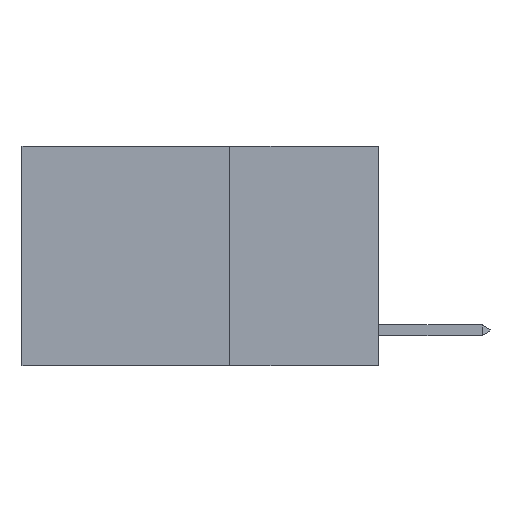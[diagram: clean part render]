
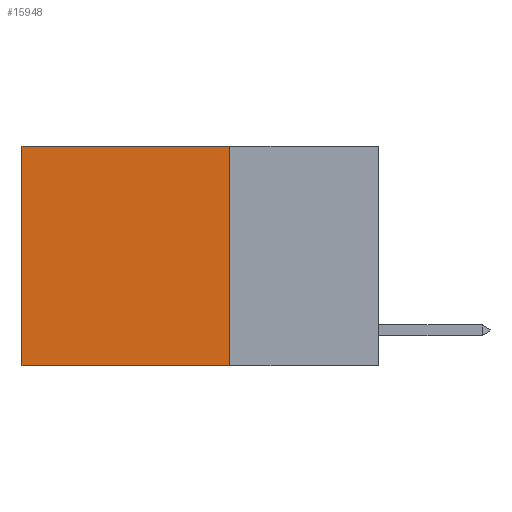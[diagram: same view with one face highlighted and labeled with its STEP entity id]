
A CAD part, left-side view. The second image highlights one B-rep face of the part: STEP entity #15948.
In plain terms, the highlighted planar face has unit normal (-1, 0, 0).
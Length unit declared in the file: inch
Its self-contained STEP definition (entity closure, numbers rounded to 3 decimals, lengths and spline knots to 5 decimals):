
#190 = CARTESIAN_POINT ( 'NONE',  ( 0.2625, 0.25, 0. ) ) ;
#525 = CARTESIAN_POINT ( 'NONE',  ( 0.2625, 0.25, -0.37 ) ) ;
#904 = VECTOR ( 'NONE', #7084, 39.37008 ) ;
#969 = EDGE_CURVE ( 'NONE', #13301, #1964, #5010, .T. ) ;
#1018 = LINE ( 'NONE', #3613, #14707 ) ;
#1738 = CARTESIAN_POINT ( 'NONE',  ( 0.2625, 0.6, -0.37 ) ) ;
#1964 = VERTEX_POINT ( 'NONE', #6426 ) ;
#2545 = PLANE ( 'NONE',  #9981 ) ;
#3000 = DIRECTION ( 'NONE',  ( 0., 0., -1. ) ) ;
#3613 = CARTESIAN_POINT ( 'NONE',  ( 0.2625, 0.6, 0. ) ) ;
#3957 = ORIENTED_EDGE ( 'NONE', *, *, #7245, .F. ) ;
#4469 = EDGE_CURVE ( 'NONE', #13301, #7602, #16827, .T. ) ;
#4696 = EDGE_CURVE ( 'NONE', #1964, #7078, #1018, .T. ) ;
#5010 = LINE ( 'NONE', #13643, #5187 ) ;
#5187 = VECTOR ( 'NONE', #16124, 39.37008 ) ;
#6251 = LINE ( 'NONE', #10553, #14449 ) ;
#6426 = CARTESIAN_POINT ( 'NONE',  ( 0.2625, 0.6, 0. ) ) ;
#6805 = DIRECTION ( 'NONE',  ( 0., 0., -1. ) ) ;
#7078 = VERTEX_POINT ( 'NONE', #1738 ) ;
#7084 = DIRECTION ( 'NONE',  ( 0., 0., -1. ) ) ;
#7245 = EDGE_CURVE ( 'NONE', #7602, #7078, #6251, .T. ) ;
#7602 = VERTEX_POINT ( 'NONE', #525 ) ;
#8506 = EDGE_LOOP ( 'NONE', ( #12573, #3957, #17761, #17839 ) ) ;
#9981 = AXIS2_PLACEMENT_3D ( 'NONE', #13843, #12629, #3000 ) ;
#10456 = DIRECTION ( 'NONE',  ( 0., 1., 0. ) ) ;
#10553 = CARTESIAN_POINT ( 'NONE',  ( 0.2625, 0.25, -0.37 ) ) ;
#12573 = ORIENTED_EDGE ( 'NONE', *, *, #4696, .T. ) ;
#12629 = DIRECTION ( 'NONE',  ( 1., 0., 0. ) ) ;
#13301 = VERTEX_POINT ( 'NONE', #13748 ) ;
#13643 = CARTESIAN_POINT ( 'NONE',  ( 0.2625, 0.25, 0. ) ) ;
#13748 = CARTESIAN_POINT ( 'NONE',  ( 0.2625, 0.25, 0. ) ) ;
#13752 = FACE_OUTER_BOUND ( 'NONE', #8506, .T. ) ;
#13843 = CARTESIAN_POINT ( 'NONE',  ( 0.2625, 0.25, 0. ) ) ;
#14449 = VECTOR ( 'NONE', #10456, 39.37008 ) ;
#14707 = VECTOR ( 'NONE', #6805, 39.37008 ) ;
#15948 = ADVANCED_FACE ( 'NONE', ( #13752 ), #2545, .F. ) ;
#16124 = DIRECTION ( 'NONE',  ( 0., 1., 0. ) ) ;
#16827 = LINE ( 'NONE', #190, #904 ) ;
#17761 = ORIENTED_EDGE ( 'NONE', *, *, #4469, .F. ) ;
#17839 = ORIENTED_EDGE ( 'NONE', *, *, #969, .T. ) ;
